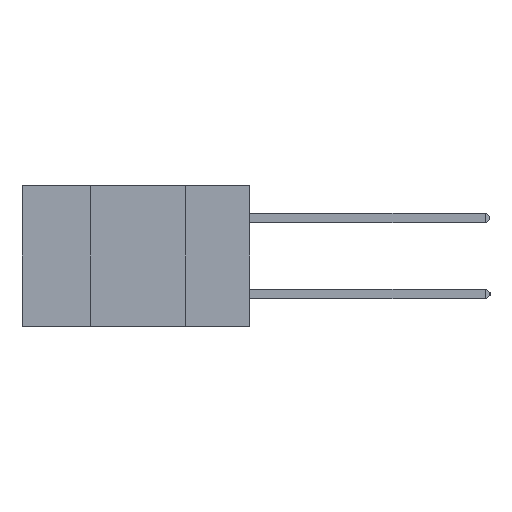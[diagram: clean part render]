
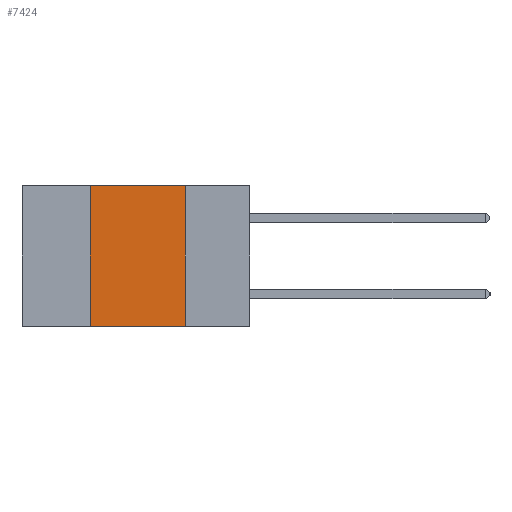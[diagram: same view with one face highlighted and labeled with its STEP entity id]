
A CAD part, left-side view. The second image highlights one B-rep face of the part: STEP entity #7424.
In plain terms, the highlighted planar face has unit normal (-1, 0, 0).
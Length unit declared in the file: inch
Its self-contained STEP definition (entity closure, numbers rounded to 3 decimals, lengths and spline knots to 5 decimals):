
#105 = VERTEX_POINT ( 'NONE', #15214 ) ;
#499 = DIRECTION ( 'NONE',  ( 0., -1., 0. ) ) ;
#668 = VECTOR ( 'NONE', #16012, 39.37008 ) ;
#992 = DIRECTION ( 'NONE',  ( 1., 0., 0. ) ) ;
#1584 = CARTESIAN_POINT ( 'NONE',  ( 0., 0.17, 0. ) ) ;
#2099 = EDGE_CURVE ( 'NONE', #11511, #105, #19187, .T. ) ;
#2206 = DIRECTION ( 'NONE',  ( 0., 0., 1. ) ) ;
#2363 = ORIENTED_EDGE ( 'NONE', *, *, #16788, .F. ) ;
#2817 = DIRECTION ( 'NONE',  ( 0., 0., -1. ) ) ;
#3678 = CARTESIAN_POINT ( 'NONE',  ( 0., 0.17, 0. ) ) ;
#4012 = LINE ( 'NONE', #7989, #12459 ) ;
#4417 = CARTESIAN_POINT ( 'NONE',  ( 0., 0.42, -0.37 ) ) ;
#5131 = EDGE_CURVE ( 'NONE', #12005, #15231, #17456, .T. ) ;
#5494 = CARTESIAN_POINT ( 'NONE',  ( 0., 0.6, -0.37 ) ) ;
#5541 = ORIENTED_EDGE ( 'NONE', *, *, #5131, .F. ) ;
#5588 = ORIENTED_EDGE ( 'NONE', *, *, #6763, .T. ) ;
#6587 = EDGE_LOOP ( 'NONE', ( #9187, #2363, #5541, #5588 ) ) ;
#6763 = EDGE_CURVE ( 'NONE', #12005, #105, #16677, .T. ) ;
#6978 = PLANE ( 'NONE',  #17176 ) ;
#7168 = FACE_OUTER_BOUND ( 'NONE', #6587, .T. ) ;
#7202 = VECTOR ( 'NONE', #2817, 39.37008 ) ;
#7424 = ADVANCED_FACE ( 'NONE', ( #7168 ), #6978, .F. ) ;
#7989 = CARTESIAN_POINT ( 'NONE',  ( 0., 0.6, 0. ) ) ;
#8482 = CARTESIAN_POINT ( 'NONE',  ( 0., 0.6, 0. ) ) ;
#9187 = ORIENTED_EDGE ( 'NONE', *, *, #2099, .F. ) ;
#11175 = CARTESIAN_POINT ( 'NONE',  ( 0., 0.42, 0. ) ) ;
#11492 = DIRECTION ( 'NONE',  ( 0., 0., -1. ) ) ;
#11511 = VERTEX_POINT ( 'NONE', #1584 ) ;
#12005 = VERTEX_POINT ( 'NONE', #4417 ) ;
#12459 = VECTOR ( 'NONE', #499, 39.37008 ) ;
#15067 = CARTESIAN_POINT ( 'NONE',  ( 0., 0.42, 0. ) ) ;
#15214 = CARTESIAN_POINT ( 'NONE',  ( 0., 0.17, -0.37 ) ) ;
#15231 = VERTEX_POINT ( 'NONE', #15067 ) ;
#16012 = DIRECTION ( 'NONE',  ( 0., -1., 0. ) ) ;
#16677 = LINE ( 'NONE', #5494, #668 ) ;
#16788 = EDGE_CURVE ( 'NONE', #15231, #11511, #4012, .T. ) ;
#17176 = AXIS2_PLACEMENT_3D ( 'NONE', #8482, #992, #11492 ) ;
#17456 = LINE ( 'NONE', #11175, #17915 ) ;
#17915 = VECTOR ( 'NONE', #2206, 39.37008 ) ;
#19187 = LINE ( 'NONE', #3678, #7202 ) ;
